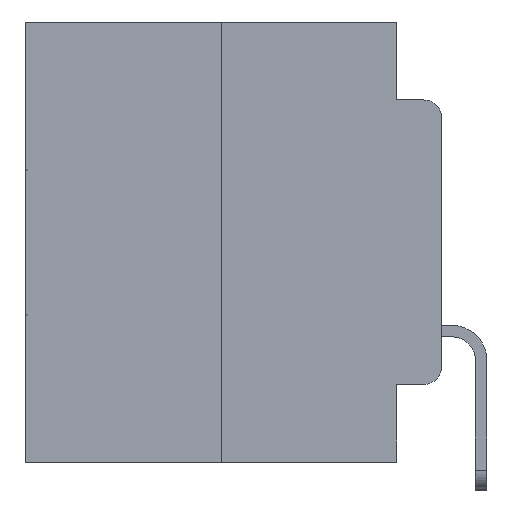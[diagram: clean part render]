
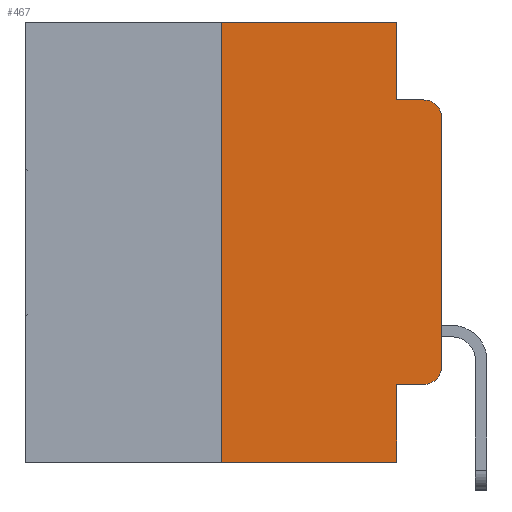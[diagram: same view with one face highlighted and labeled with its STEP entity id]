
A CAD part, left-side view. The second image highlights one B-rep face of the part: STEP entity #467.
In plain terms, the highlighted planar face has unit normal (-1, 0, 0).
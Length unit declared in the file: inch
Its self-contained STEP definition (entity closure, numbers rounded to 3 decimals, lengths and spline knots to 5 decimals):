
#53 = CIRCLE ( 'NONE', #21203, 0.02 ) ;
#213 = DIRECTION ( 'NONE',  ( 0., 0., 1. ) ) ;
#311 = ORIENTED_EDGE ( 'NONE', *, *, #15738, .T. ) ;
#467 = ADVANCED_FACE ( 'NONE', ( #19944 ), #4127, .F. ) ;
#1904 = ORIENTED_EDGE ( 'NONE', *, *, #16847, .F. ) ;
#2903 = EDGE_CURVE ( 'NONE', #15190, #12309, #53, .T. ) ;
#3136 = LINE ( 'NONE', #24272, #26258 ) ;
#3168 = EDGE_CURVE ( 'NONE', #3999, #12924, #3713, .T. ) ;
#3201 = VERTEX_POINT ( 'NONE', #7299 ) ;
#3527 = AXIS2_PLACEMENT_3D ( 'NONE', #23423, #10131, #25612 ) ;
#3625 = CARTESIAN_POINT ( 'NONE',  ( 0., 0., 0. ) ) ;
#3713 = LINE ( 'NONE', #25669, #5174 ) ;
#3999 = VERTEX_POINT ( 'NONE', #5703 ) ;
#4127 = PLANE ( 'NONE',  #20291 ) ;
#4162 = CARTESIAN_POINT ( 'NONE',  ( 0., 0.02, -0.4115 ) ) ;
#4473 = CARTESIAN_POINT ( 'NONE',  ( 0., 0.051, -0.4115 ) ) ;
#4582 = VECTOR ( 'NONE', #28841, 39.37008 ) ;
#5112 = ORIENTED_EDGE ( 'NONE', *, *, #3168, .T. ) ;
#5174 = VECTOR ( 'NONE', #14547, 39.37008 ) ;
#5342 = LINE ( 'NONE', #17919, #4582 ) ;
#5703 = CARTESIAN_POINT ( 'NONE',  ( 0., 0.25, -0.5 ) ) ;
#6028 = EDGE_LOOP ( 'NONE', ( #24306, #10476, #12919, #21530, #24602, #18165, #5112, #1904, #6516, #311 ) ) ;
#6106 = LINE ( 'NONE', #23205, #11424 ) ;
#6172 = VECTOR ( 'NONE', #25096, 39.37008 ) ;
#6516 = ORIENTED_EDGE ( 'NONE', *, *, #17770, .T. ) ;
#7299 = CARTESIAN_POINT ( 'NONE',  ( 0., 0.051, -0.0885 ) ) ;
#8219 = VERTEX_POINT ( 'NONE', #13266 ) ;
#8358 = CARTESIAN_POINT ( 'NONE',  ( 0., 0.051, -0.4115 ) ) ;
#8392 = CARTESIAN_POINT ( 'NONE',  ( 0., 0.25, 0. ) ) ;
#9464 = VERTEX_POINT ( 'NONE', #4162 ) ;
#9950 = VECTOR ( 'NONE', #15006, 39.37008 ) ;
#10046 = EDGE_CURVE ( 'NONE', #3201, #12309, #5342, .T. ) ;
#10131 = DIRECTION ( 'NONE',  ( -1., 0., 0. ) ) ;
#10329 = VERTEX_POINT ( 'NONE', #19045 ) ;
#10476 = ORIENTED_EDGE ( 'NONE', *, *, #2903, .T. ) ;
#11424 = VECTOR ( 'NONE', #14440, 39.37008 ) ;
#11736 = CARTESIAN_POINT ( 'NONE',  ( 0., 0.25, 0. ) ) ;
#11908 = CARTESIAN_POINT ( 'NONE',  ( 0., 0.051, 0. ) ) ;
#12309 = VERTEX_POINT ( 'NONE', #19623 ) ;
#12919 = ORIENTED_EDGE ( 'NONE', *, *, #10046, .F. ) ;
#12924 = VERTEX_POINT ( 'NONE', #15249 ) ;
#12942 = DIRECTION ( 'NONE',  ( 0., -1., 0. ) ) ;
#13197 = DIRECTION ( 'NONE',  ( 0., 0., -1. ) ) ;
#13266 = CARTESIAN_POINT ( 'NONE',  ( 0., 0.051, 0. ) ) ;
#14020 = CIRCLE ( 'NONE', #3527, 0.02 ) ;
#14440 = DIRECTION ( 'NONE',  ( 0., -1., 0. ) ) ;
#14547 = DIRECTION ( 'NONE',  ( 0., -1., 0. ) ) ;
#15006 = DIRECTION ( 'NONE',  ( 0., 0., 1. ) ) ;
#15190 = VERTEX_POINT ( 'NONE', #19445 ) ;
#15249 = CARTESIAN_POINT ( 'NONE',  ( 0., 0.051, -0.5 ) ) ;
#15661 = DIRECTION ( 'NONE',  ( 0., 0., -1. ) ) ;
#15738 = EDGE_CURVE ( 'NONE', #9464, #10329, #14020, .T. ) ;
#16092 = VERTEX_POINT ( 'NONE', #4473 ) ;
#16811 = CARTESIAN_POINT ( 'NONE',  ( 0., 0.02, -0.1085 ) ) ;
#16847 = EDGE_CURVE ( 'NONE', #16092, #12924, #28994, .T. ) ;
#16968 = VECTOR ( 'NONE', #213, 39.37008 ) ;
#17374 = LINE ( 'NONE', #8358, #28273 ) ;
#17770 = EDGE_CURVE ( 'NONE', #16092, #9464, #17374, .T. ) ;
#17919 = CARTESIAN_POINT ( 'NONE',  ( 0., 0.051, -0.0885 ) ) ;
#18165 = ORIENTED_EDGE ( 'NONE', *, *, #19422, .F. ) ;
#18493 = EDGE_CURVE ( 'NONE', #8219, #3201, #3136, .T. ) ;
#19045 = CARTESIAN_POINT ( 'NONE',  ( 0., 0., -0.3915 ) ) ;
#19422 = EDGE_CURVE ( 'NONE', #3999, #24792, #28544, .T. ) ;
#19445 = CARTESIAN_POINT ( 'NONE',  ( 0., 0., -0.1085 ) ) ;
#19623 = CARTESIAN_POINT ( 'NONE',  ( 0., 0.02, -0.0885 ) ) ;
#19944 = FACE_OUTER_BOUND ( 'NONE', #6028, .T. ) ;
#20291 = AXIS2_PLACEMENT_3D ( 'NONE', #27555, #27420, #13197 ) ;
#21203 = AXIS2_PLACEMENT_3D ( 'NONE', #16811, #25539, #15661 ) ;
#21208 = EDGE_CURVE ( 'NONE', #10329, #15190, #28244, .T. ) ;
#21530 = ORIENTED_EDGE ( 'NONE', *, *, #18493, .F. ) ;
#23205 = CARTESIAN_POINT ( 'NONE',  ( 0., 0.473, 0. ) ) ;
#23423 = CARTESIAN_POINT ( 'NONE',  ( 0., 0.02, -0.3915 ) ) ;
#24272 = CARTESIAN_POINT ( 'NONE',  ( 0., 0.051, 0. ) ) ;
#24306 = ORIENTED_EDGE ( 'NONE', *, *, #21208, .T. ) ;
#24602 = ORIENTED_EDGE ( 'NONE', *, *, #26233, .F. ) ;
#24792 = VERTEX_POINT ( 'NONE', #8392 ) ;
#25096 = DIRECTION ( 'NONE',  ( 0., 0., -1. ) ) ;
#25539 = DIRECTION ( 'NONE',  ( -1., 0., 0. ) ) ;
#25612 = DIRECTION ( 'NONE',  ( 0., 0., -1. ) ) ;
#25669 = CARTESIAN_POINT ( 'NONE',  ( 0., 0.473, -0.5 ) ) ;
#26233 = EDGE_CURVE ( 'NONE', #24792, #8219, #6106, .T. ) ;
#26258 = VECTOR ( 'NONE', #26358, 39.37008 ) ;
#26358 = DIRECTION ( 'NONE',  ( 0., 0., -1. ) ) ;
#27420 = DIRECTION ( 'NONE',  ( 1., 0., 0. ) ) ;
#27555 = CARTESIAN_POINT ( 'NONE',  ( 0., 0.473, 0. ) ) ;
#28244 = LINE ( 'NONE', #3625, #9950 ) ;
#28273 = VECTOR ( 'NONE', #12942, 39.37008 ) ;
#28544 = LINE ( 'NONE', #11736, #16968 ) ;
#28841 = DIRECTION ( 'NONE',  ( 0., -1., 0. ) ) ;
#28994 = LINE ( 'NONE', #11908, #6172 ) ;
